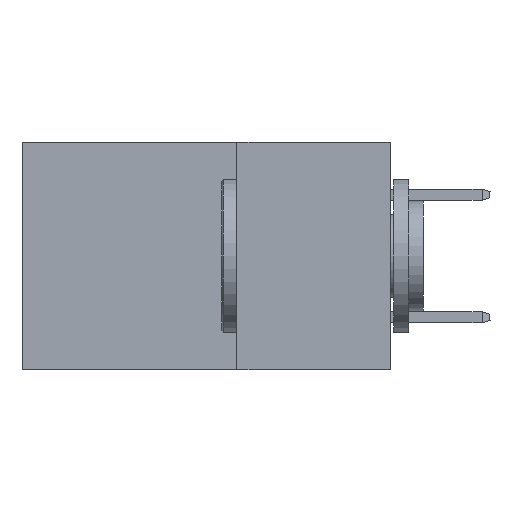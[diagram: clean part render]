
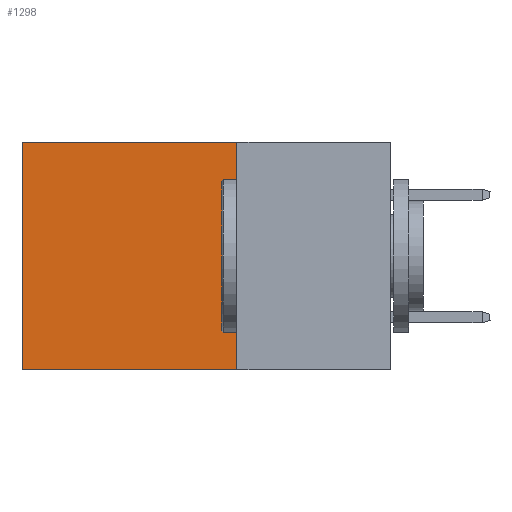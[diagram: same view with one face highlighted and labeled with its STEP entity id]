
A CAD part, left-side view. The second image highlights one B-rep face of the part: STEP entity #1298.
In plain terms, the highlighted planar face has unit normal (-1, 0, 0).
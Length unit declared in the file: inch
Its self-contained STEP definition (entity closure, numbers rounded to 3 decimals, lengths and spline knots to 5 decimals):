
#1298 = ADVANCED_FACE ( 'NONE', ( #13164 ), #12335, .F. ) ;
#1373 = CARTESIAN_POINT ( 'NONE',  ( 0.2875, 0.25, 0. ) ) ;
#2349 = EDGE_CURVE ( 'NONE', #22519, #9946, #11467, .T. ) ;
#2360 = ORIENTED_EDGE ( 'NONE', *, *, #2349, .F. ) ;
#3602 = VECTOR ( 'NONE', #4646, 39.37008 ) ;
#3952 = ORIENTED_EDGE ( 'NONE', *, *, #7765, .T. ) ;
#4171 = CARTESIAN_POINT ( 'NONE',  ( 0.2875, 0.25, 0. ) ) ;
#4423 = VECTOR ( 'NONE', #15854, 39.37008 ) ;
#4481 = EDGE_LOOP ( 'NONE', ( #3952, #10468, #2360, #14963 ) ) ;
#4646 = DIRECTION ( 'NONE',  ( 0., 1., 0. ) ) ;
#4660 = CARTESIAN_POINT ( 'NONE',  ( 0.2875, 0.6, -0.37 ) ) ;
#6024 = CARTESIAN_POINT ( 'NONE',  ( 0.2875, 0.25, -0.37 ) ) ;
#6214 = CARTESIAN_POINT ( 'NONE',  ( 0.2875, 0.6, 0. ) ) ;
#6801 = DIRECTION ( 'NONE',  ( 0., 0., -1. ) ) ;
#7032 = VECTOR ( 'NONE', #18319, 39.37008 ) ;
#7057 = CARTESIAN_POINT ( 'NONE',  ( 0.2875, 0.25, 0. ) ) ;
#7315 = LINE ( 'NONE', #6024, #7032 ) ;
#7715 = VECTOR ( 'NONE', #9738, 39.37008 ) ;
#7765 = EDGE_CURVE ( 'NONE', #20918, #21673, #18916, .T. ) ;
#8665 = AXIS2_PLACEMENT_3D ( 'NONE', #1373, #17552, #6801 ) ;
#9738 = DIRECTION ( 'NONE',  ( 0., 0., -1. ) ) ;
#9941 = CARTESIAN_POINT ( 'NONE',  ( 0.2875, 0.25, -0.37 ) ) ;
#9946 = VERTEX_POINT ( 'NONE', #9941 ) ;
#10468 = ORIENTED_EDGE ( 'NONE', *, *, #16182, .F. ) ;
#11467 = LINE ( 'NONE', #7057, #4423 ) ;
#11510 = EDGE_CURVE ( 'NONE', #22519, #20918, #22434, .T. ) ;
#12335 = PLANE ( 'NONE',  #8665 ) ;
#13164 = FACE_OUTER_BOUND ( 'NONE', #4481, .T. ) ;
#14963 = ORIENTED_EDGE ( 'NONE', *, *, #11510, .T. ) ;
#15416 = CARTESIAN_POINT ( 'NONE',  ( 0.2875, 0.6, 0. ) ) ;
#15854 = DIRECTION ( 'NONE',  ( 0., 0., -1. ) ) ;
#16182 = EDGE_CURVE ( 'NONE', #9946, #21673, #7315, .T. ) ;
#17552 = DIRECTION ( 'NONE',  ( 1., 0., 0. ) ) ;
#18319 = DIRECTION ( 'NONE',  ( 0., 1., 0. ) ) ;
#18916 = LINE ( 'NONE', #6214, #7715 ) ;
#20918 = VERTEX_POINT ( 'NONE', #15416 ) ;
#21523 = CARTESIAN_POINT ( 'NONE',  ( 0.2875, 0.25, 0. ) ) ;
#21673 = VERTEX_POINT ( 'NONE', #4660 ) ;
#22434 = LINE ( 'NONE', #4171, #3602 ) ;
#22519 = VERTEX_POINT ( 'NONE', #21523 ) ;
